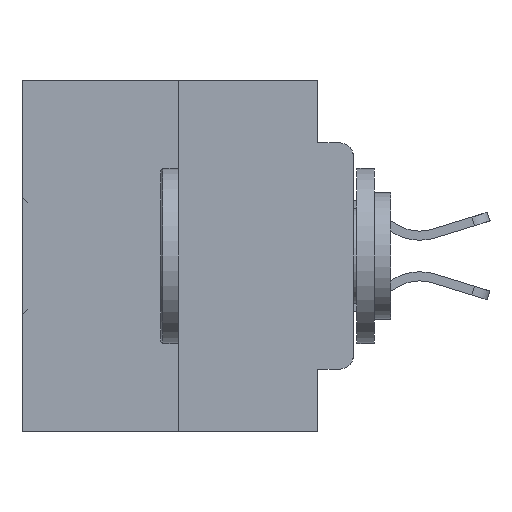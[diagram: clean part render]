
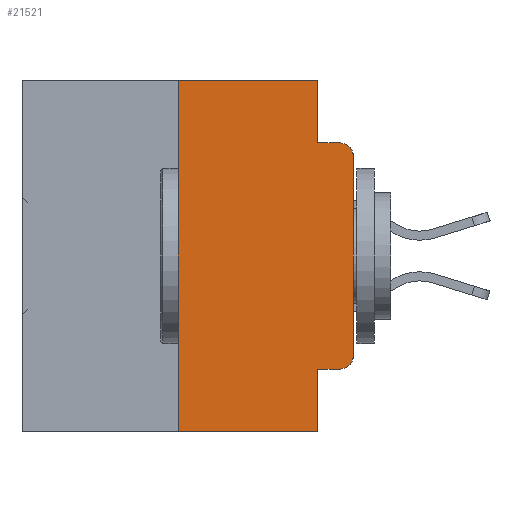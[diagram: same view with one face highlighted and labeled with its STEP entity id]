
A CAD part, left-side view. The second image highlights one B-rep face of the part: STEP entity #21521.
In plain terms, the highlighted planar face has unit normal (-1, 0, 0).
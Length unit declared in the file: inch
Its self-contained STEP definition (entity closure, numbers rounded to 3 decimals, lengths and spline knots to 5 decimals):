
#98 = DIRECTION ( 'NONE',  ( 0., -1., 0. ) ) ;
#514 = ORIENTED_EDGE ( 'NONE', *, *, #29914, .T. ) ;
#781 = CARTESIAN_POINT ( 'NONE',  ( 0., 0.02, -0.0885 ) ) ;
#782 = CARTESIAN_POINT ( 'NONE',  ( 0., 0.25, 0. ) ) ;
#1465 = VERTEX_POINT ( 'NONE', #2732 ) ;
#1533 = ORIENTED_EDGE ( 'NONE', *, *, #3829, .F. ) ;
#1983 = ORIENTED_EDGE ( 'NONE', *, *, #9798, .T. ) ;
#2018 = DIRECTION ( 'NONE',  ( 0., 0., -1. ) ) ;
#2151 = ORIENTED_EDGE ( 'NONE', *, *, #19804, .T. ) ;
#2732 = CARTESIAN_POINT ( 'NONE',  ( 0., 0.051, -0.0885 ) ) ;
#3651 = DIRECTION ( 'NONE',  ( 1., 0., 0. ) ) ;
#3829 = EDGE_CURVE ( 'NONE', #7809, #21338, #19727, .T. ) ;
#4907 = CARTESIAN_POINT ( 'NONE',  ( 0., 0., -0.3915 ) ) ;
#5046 = VERTEX_POINT ( 'NONE', #4907 ) ;
#7809 = VERTEX_POINT ( 'NONE', #21863 ) ;
#8394 = VECTOR ( 'NONE', #11771, 39.37008 ) ;
#8703 = VERTEX_POINT ( 'NONE', #781 ) ;
#8798 = VECTOR ( 'NONE', #30729, 39.37008 ) ;
#8870 = VERTEX_POINT ( 'NONE', #23126 ) ;
#9798 = EDGE_CURVE ( 'NONE', #7809, #20507, #27707, .T. ) ;
#9963 = CARTESIAN_POINT ( 'NONE',  ( 0., 0.25, -0.5 ) ) ;
#10866 = VERTEX_POINT ( 'NONE', #34705 ) ;
#11194 = DIRECTION ( 'NONE',  ( 0., -1., 0. ) ) ;
#11195 = CARTESIAN_POINT ( 'NONE',  ( 0., 0.02, -0.1085 ) ) ;
#11220 = DIRECTION ( 'NONE',  ( 0., -1., 0. ) ) ;
#11771 = DIRECTION ( 'NONE',  ( 0., 0., 1. ) ) ;
#13963 = DIRECTION ( 'NONE',  ( 0., 0., -1. ) ) ;
#14427 = DIRECTION ( 'NONE',  ( 0., 0., -1. ) ) ;
#15198 = CARTESIAN_POINT ( 'NONE',  ( 0., 0.051, 0. ) ) ;
#16088 = LINE ( 'NONE', #22632, #8798 ) ;
#16701 = CIRCLE ( 'NONE', #33981, 0.02 ) ;
#16748 = AXIS2_PLACEMENT_3D ( 'NONE', #17280, #3651, #22610 ) ;
#16863 = CIRCLE ( 'NONE', #32156, 0.02 ) ;
#17100 = CARTESIAN_POINT ( 'NONE',  ( 0., 0.051, 0. ) ) ;
#17280 = CARTESIAN_POINT ( 'NONE',  ( 0., 0.473, 0. ) ) ;
#17392 = LINE ( 'NONE', #782, #8394 ) ;
#17632 = ORIENTED_EDGE ( 'NONE', *, *, #18897, .T. ) ;
#17771 = DIRECTION ( 'NONE',  ( 0., -1., 0. ) ) ;
#18386 = DIRECTION ( 'NONE',  ( -1., 0., 0. ) ) ;
#18793 = VECTOR ( 'NONE', #11194, 39.37008 ) ;
#18897 = EDGE_CURVE ( 'NONE', #5046, #8870, #16088, .T. ) ;
#19242 = ORIENTED_EDGE ( 'NONE', *, *, #21992, .T. ) ;
#19613 = VECTOR ( 'NONE', #17771, 39.37008 ) ;
#19626 = LINE ( 'NONE', #27272, #18793 ) ;
#19727 = LINE ( 'NONE', #32698, #25143 ) ;
#19758 = VECTOR ( 'NONE', #11220, 39.37008 ) ;
#19804 = EDGE_CURVE ( 'NONE', #20507, #5046, #16863, .T. ) ;
#20130 = EDGE_CURVE ( 'NONE', #33939, #1465, #20992, .T. ) ;
#20507 = VERTEX_POINT ( 'NONE', #26198 ) ;
#20992 = LINE ( 'NONE', #17100, #27271 ) ;
#21338 = VERTEX_POINT ( 'NONE', #24487 ) ;
#21521 = ADVANCED_FACE ( 'NONE', ( #31779 ), #25190, .F. ) ;
#21768 = ORIENTED_EDGE ( 'NONE', *, *, #28987, .F. ) ;
#21863 = CARTESIAN_POINT ( 'NONE',  ( 0., 0.051, -0.4115 ) ) ;
#21992 = EDGE_CURVE ( 'NONE', #8870, #8703, #16701, .T. ) ;
#22488 = VECTOR ( 'NONE', #98, 39.37008 ) ;
#22610 = DIRECTION ( 'NONE',  ( 0., 0., -1. ) ) ;
#22632 = CARTESIAN_POINT ( 'NONE',  ( 0., 0., 0. ) ) ;
#23126 = CARTESIAN_POINT ( 'NONE',  ( 0., 0., -0.1085 ) ) ;
#23428 = ORIENTED_EDGE ( 'NONE', *, *, #20130, .F. ) ;
#23462 = ORIENTED_EDGE ( 'NONE', *, *, #28416, .F. ) ;
#24487 = CARTESIAN_POINT ( 'NONE',  ( 0., 0.051, -0.5 ) ) ;
#24703 = CARTESIAN_POINT ( 'NONE',  ( 0., 0.051, -0.4115 ) ) ;
#24900 = EDGE_CURVE ( 'NONE', #26841, #10866, #17392, .T. ) ;
#25143 = VECTOR ( 'NONE', #31783, 39.37008 ) ;
#25190 = PLANE ( 'NONE',  #16748 ) ;
#26198 = CARTESIAN_POINT ( 'NONE',  ( 0., 0.02, -0.4115 ) ) ;
#26841 = VERTEX_POINT ( 'NONE', #9963 ) ;
#27154 = CARTESIAN_POINT ( 'NONE',  ( 0., 0.051, -0.0885 ) ) ;
#27271 = VECTOR ( 'NONE', #14427, 39.37008 ) ;
#27272 = CARTESIAN_POINT ( 'NONE',  ( 0., 0.473, 0. ) ) ;
#27707 = LINE ( 'NONE', #24703, #19758 ) ;
#28093 = ORIENTED_EDGE ( 'NONE', *, *, #24900, .F. ) ;
#28416 = EDGE_CURVE ( 'NONE', #10866, #33939, #19626, .T. ) ;
#28987 = EDGE_CURVE ( 'NONE', #1465, #8703, #30462, .T. ) ;
#29876 = EDGE_LOOP ( 'NONE', ( #17632, #19242, #21768, #23428, #23462, #28093, #514, #1533, #1983, #2151 ) ) ;
#29914 = EDGE_CURVE ( 'NONE', #26841, #21338, #33832, .T. ) ;
#29980 = DIRECTION ( 'NONE',  ( -1., 0., 0. ) ) ;
#30462 = LINE ( 'NONE', #27154, #22488 ) ;
#30729 = DIRECTION ( 'NONE',  ( 0., 0., 1. ) ) ;
#30853 = CARTESIAN_POINT ( 'NONE',  ( 0., 0.473, -0.5 ) ) ;
#31779 = FACE_OUTER_BOUND ( 'NONE', #29876, .T. ) ;
#31783 = DIRECTION ( 'NONE',  ( 0., 0., -1. ) ) ;
#32156 = AXIS2_PLACEMENT_3D ( 'NONE', #34392, #18386, #2018 ) ;
#32698 = CARTESIAN_POINT ( 'NONE',  ( 0., 0.051, 0. ) ) ;
#33832 = LINE ( 'NONE', #30853, #19613 ) ;
#33939 = VERTEX_POINT ( 'NONE', #15198 ) ;
#33981 = AXIS2_PLACEMENT_3D ( 'NONE', #11195, #29980, #13963 ) ;
#34392 = CARTESIAN_POINT ( 'NONE',  ( 0., 0.02, -0.3915 ) ) ;
#34705 = CARTESIAN_POINT ( 'NONE',  ( 0., 0.25, 0. ) ) ;
